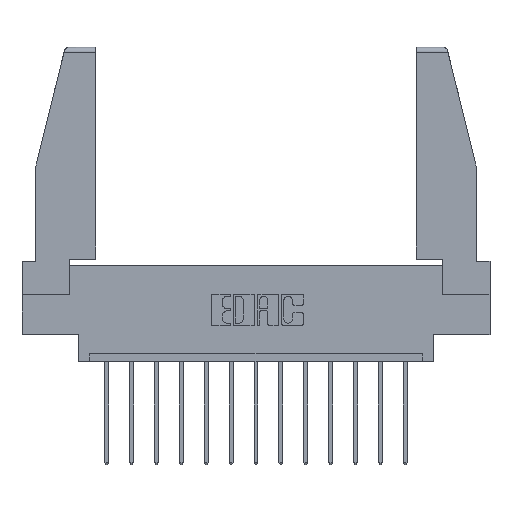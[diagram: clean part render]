
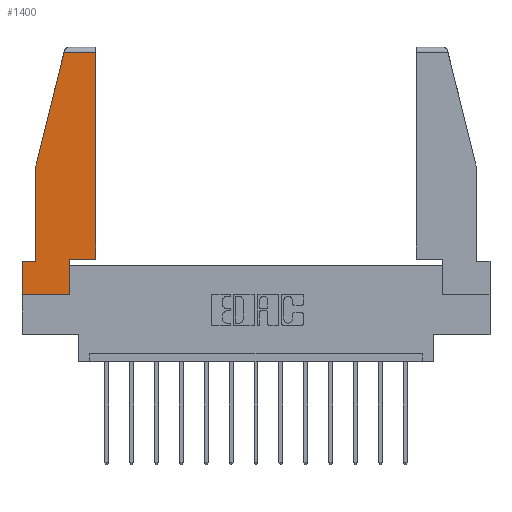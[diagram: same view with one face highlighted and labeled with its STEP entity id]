
A CAD part, top view. The second image highlights one B-rep face of the part: STEP entity #1400.
In plain terms, the highlighted planar face has unit normal (0, 0, 1).
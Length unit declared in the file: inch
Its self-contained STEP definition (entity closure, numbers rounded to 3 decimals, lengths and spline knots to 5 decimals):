
#89 = EDGE_CURVE ( 'NONE', #7742, #12126, #15388, .T. ) ;
#108 = EDGE_CURVE ( 'NONE', #7166, #1098, #14245, .T. ) ;
#110 = VECTOR ( 'NONE', #6683, 39.37008 ) ;
#164 = VECTOR ( 'NONE', #494, 39.37008 ) ;
#317 = VECTOR ( 'NONE', #5509, 39.37008 ) ;
#400 = DIRECTION ( 'NONE',  ( 0., -1., 0. ) ) ;
#494 = DIRECTION ( 'NONE',  ( -0.239, -0.971, 0. ) ) ;
#553 = CARTESIAN_POINT ( 'NONE',  ( 0., 0.21, 0. ) ) ;
#1098 = VERTEX_POINT ( 'NONE', #2921 ) ;
#1354 = ORIENTED_EDGE ( 'NONE', *, *, #13039, .T. ) ;
#1400 = ADVANCED_FACE ( 'NONE', ( #5288 ), #3235, .T. ) ;
#1482 = ORIENTED_EDGE ( 'NONE', *, *, #12066, .T. ) ;
#2152 = LINE ( 'NONE', #10084, #15864 ) ;
#2431 = DIRECTION ( 'NONE',  ( 0., 1., 0. ) ) ;
#2546 = CARTESIAN_POINT ( 'NONE',  ( 0.297, 0.223, 0. ) ) ;
#2921 = CARTESIAN_POINT ( 'NONE',  ( 0., 0., 0. ) ) ;
#3235 = PLANE ( 'NONE',  #14002 ) ;
#3848 = VECTOR ( 'NONE', #2431, 39.37008 ) ;
#3999 = CARTESIAN_POINT ( 'NONE',  ( 0.2636, 1.52, 0. ) ) ;
#4160 = EDGE_CURVE ( 'NONE', #12126, #14876, #12812, .T. ) ;
#5288 = FACE_OUTER_BOUND ( 'NONE', #7268, .T. ) ;
#5319 = VECTOR ( 'NONE', #15952, 39.37008 ) ;
#5443 = CARTESIAN_POINT ( 'NONE',  ( 0.297, 0., 0. ) ) ;
#5469 = CARTESIAN_POINT ( 'NONE',  ( 0.297, 0.223, 0. ) ) ;
#5481 = CARTESIAN_POINT ( 'NONE',  ( 0.271, 1.55, 0. ) ) ;
#5509 = DIRECTION ( 'NONE',  ( 1., 0., 0. ) ) ;
#5545 = CARTESIAN_POINT ( 'NONE',  ( 0.086, 0.8, 0. ) ) ;
#5789 = ORIENTED_EDGE ( 'NONE', *, *, #7988, .T. ) ;
#6211 = CARTESIAN_POINT ( 'NONE',  ( 0.461, 0.223, 0. ) ) ;
#6224 = VECTOR ( 'NONE', #14436, 39.37008 ) ;
#6683 = DIRECTION ( 'NONE',  ( 0., 1., 0. ) ) ;
#6729 = CARTESIAN_POINT ( 'NONE',  ( 0.461, 0.223, 0. ) ) ;
#7166 = VERTEX_POINT ( 'NONE', #8766 ) ;
#7174 = DIRECTION ( 'NONE',  ( 0., 0., 1. ) ) ;
#7268 = EDGE_LOOP ( 'NONE', ( #10684, #1482, #1354, #11780, #15407, #11752, #5789, #15079, #9663 ) ) ;
#7742 = VERTEX_POINT ( 'NONE', #10015 ) ;
#7840 = CARTESIAN_POINT ( 'NONE',  ( 0., 0.21, 0. ) ) ;
#7954 = LINE ( 'NONE', #5481, #164 ) ;
#7988 = EDGE_CURVE ( 'NONE', #1098, #7742, #15410, .T. ) ;
#8365 = CARTESIAN_POINT ( 'NONE',  ( 0.461, 1.52, 0. ) ) ;
#8451 = CARTESIAN_POINT ( 'NONE',  ( 0.086, 0.8, 0. ) ) ;
#8766 = CARTESIAN_POINT ( 'NONE',  ( 0., 0.21, 0. ) ) ;
#8791 = EDGE_CURVE ( 'NONE', #9146, #7166, #12091, .T. ) ;
#8812 = VERTEX_POINT ( 'NONE', #5545 ) ;
#9146 = VERTEX_POINT ( 'NONE', #15842 ) ;
#9253 = DIRECTION ( 'NONE',  ( -1., 0., 0. ) ) ;
#9322 = LINE ( 'NONE', #6211, #3848 ) ;
#9663 = ORIENTED_EDGE ( 'NONE', *, *, #4160, .T. ) ;
#9865 = VERTEX_POINT ( 'NONE', #8365 ) ;
#10015 = CARTESIAN_POINT ( 'NONE',  ( 0.297, 0., 0. ) ) ;
#10084 = CARTESIAN_POINT ( 'NONE',  ( 0., 1.52, 0. ) ) ;
#10201 = DIRECTION ( 'NONE',  ( -1., 0., 0. ) ) ;
#10573 = VECTOR ( 'NONE', #9253, 39.37008 ) ;
#10684 = ORIENTED_EDGE ( 'NONE', *, *, #12398, .T. ) ;
#11752 = ORIENTED_EDGE ( 'NONE', *, *, #108, .T. ) ;
#11780 = ORIENTED_EDGE ( 'NONE', *, *, #14149, .T. ) ;
#12040 = DIRECTION ( 'NONE',  ( 1., 0., 0. ) ) ;
#12066 = EDGE_CURVE ( 'NONE', #9865, #12172, #2152, .T. ) ;
#12091 = LINE ( 'NONE', #553, #10573 ) ;
#12126 = VERTEX_POINT ( 'NONE', #2546 ) ;
#12172 = VERTEX_POINT ( 'NONE', #3999 ) ;
#12398 = EDGE_CURVE ( 'NONE', #14876, #9865, #9322, .T. ) ;
#12654 = LINE ( 'NONE', #8451, #5319 ) ;
#12812 = LINE ( 'NONE', #5469, #6224 ) ;
#13039 = EDGE_CURVE ( 'NONE', #12172, #8812, #7954, .T. ) ;
#13131 = CARTESIAN_POINT ( 'NONE',  ( 0., 0., 0. ) ) ;
#13949 = CARTESIAN_POINT ( 'NONE',  ( 0., 0., 0. ) ) ;
#14002 = AXIS2_PLACEMENT_3D ( 'NONE', #13131, #7174, #12040 ) ;
#14149 = EDGE_CURVE ( 'NONE', #8812, #9146, #12654, .T. ) ;
#14245 = LINE ( 'NONE', #7840, #14993 ) ;
#14436 = DIRECTION ( 'NONE',  ( 1., 0., 0. ) ) ;
#14876 = VERTEX_POINT ( 'NONE', #6729 ) ;
#14993 = VECTOR ( 'NONE', #400, 39.37008 ) ;
#15079 = ORIENTED_EDGE ( 'NONE', *, *, #89, .T. ) ;
#15388 = LINE ( 'NONE', #5443, #110 ) ;
#15407 = ORIENTED_EDGE ( 'NONE', *, *, #8791, .T. ) ;
#15410 = LINE ( 'NONE', #13949, #317 ) ;
#15842 = CARTESIAN_POINT ( 'NONE',  ( 0.086, 0.21, 0. ) ) ;
#15864 = VECTOR ( 'NONE', #10201, 39.37008 ) ;
#15952 = DIRECTION ( 'NONE',  ( 0., -1., 0. ) ) ;
